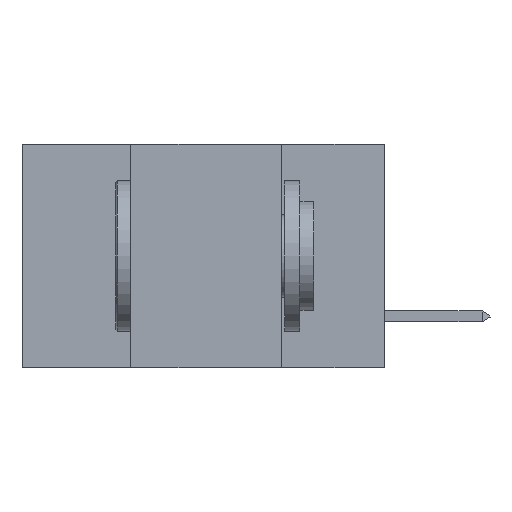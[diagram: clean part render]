
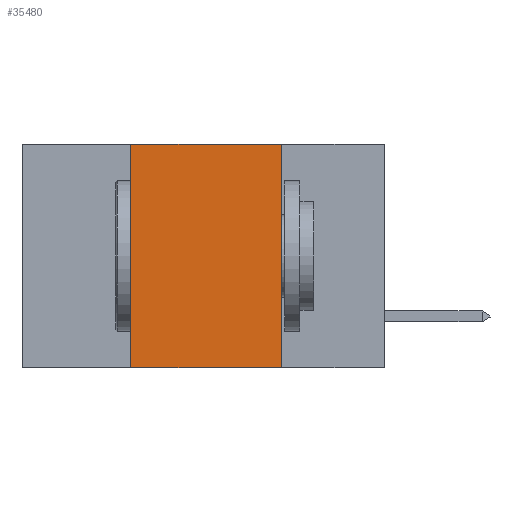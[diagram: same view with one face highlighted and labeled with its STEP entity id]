
A CAD part, left-side view. The second image highlights one B-rep face of the part: STEP entity #35480.
In plain terms, the highlighted planar face has unit normal (-1, 0, 0).
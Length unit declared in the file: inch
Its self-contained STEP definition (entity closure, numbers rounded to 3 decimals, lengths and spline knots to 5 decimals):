
#1150 = CARTESIAN_POINT ( 'NONE',  ( 0., 0.17, -0.37 ) ) ;
#1853 = CARTESIAN_POINT ( 'NONE',  ( 0., 0.42, 0. ) ) ;
#5562 = ORIENTED_EDGE ( 'NONE', *, *, #40684, .F. ) ;
#9943 = VECTOR ( 'NONE', #13408, 39.37008 ) ;
#10858 = DIRECTION ( 'NONE',  ( 0., -1., 0. ) ) ;
#11159 = ORIENTED_EDGE ( 'NONE', *, *, #45193, .T. ) ;
#12161 = DIRECTION ( 'NONE',  ( 0., -1., 0. ) ) ;
#12450 = EDGE_LOOP ( 'NONE', ( #5562, #14109, #42542, #11159 ) ) ;
#12454 = LINE ( 'NONE', #26437, #38988 ) ;
#12460 = CARTESIAN_POINT ( 'NONE',  ( 0., 0.6, 0. ) ) ;
#12589 = VERTEX_POINT ( 'NONE', #1150 ) ;
#13408 = DIRECTION ( 'NONE',  ( 0., 0., 1. ) ) ;
#13630 = VECTOR ( 'NONE', #12161, 39.37008 ) ;
#14109 = ORIENTED_EDGE ( 'NONE', *, *, #49645, .F. ) ;
#15877 = FACE_OUTER_BOUND ( 'NONE', #12450, .T. ) ;
#19212 = LINE ( 'NONE', #19946, #13630 ) ;
#19946 = CARTESIAN_POINT ( 'NONE',  ( 0., 0.6, -0.37 ) ) ;
#21953 = AXIS2_PLACEMENT_3D ( 'NONE', #12460, #40065, #24423 ) ;
#24423 = DIRECTION ( 'NONE',  ( 0., 0., -1. ) ) ;
#24601 = LINE ( 'NONE', #28162, #37528 ) ;
#26326 = VERTEX_POINT ( 'NONE', #37437 ) ;
#26437 = CARTESIAN_POINT ( 'NONE',  ( 0., 0.6, 0. ) ) ;
#28162 = CARTESIAN_POINT ( 'NONE',  ( 0., 0.17, 0. ) ) ;
#35480 = ADVANCED_FACE ( 'NONE', ( #15877 ), #36307, .F. ) ;
#36307 = PLANE ( 'NONE',  #21953 ) ;
#36536 = CARTESIAN_POINT ( 'NONE',  ( 0., 0.17, 0. ) ) ;
#37437 = CARTESIAN_POINT ( 'NONE',  ( 0., 0.42, 0. ) ) ;
#37528 = VECTOR ( 'NONE', #39824, 39.37008 ) ;
#38988 = VECTOR ( 'NONE', #10858, 39.37008 ) ;
#39824 = DIRECTION ( 'NONE',  ( 0., 0., -1. ) ) ;
#40065 = DIRECTION ( 'NONE',  ( 1., 0., 0. ) ) ;
#40684 = EDGE_CURVE ( 'NONE', #46856, #12589, #24601, .T. ) ;
#40964 = VERTEX_POINT ( 'NONE', #49259 ) ;
#42542 = ORIENTED_EDGE ( 'NONE', *, *, #50031, .F. ) ;
#45193 = EDGE_CURVE ( 'NONE', #40964, #12589, #19212, .T. ) ;
#46856 = VERTEX_POINT ( 'NONE', #36536 ) ;
#48759 = LINE ( 'NONE', #1853, #9943 ) ;
#49259 = CARTESIAN_POINT ( 'NONE',  ( 0., 0.42, -0.37 ) ) ;
#49645 = EDGE_CURVE ( 'NONE', #26326, #46856, #12454, .T. ) ;
#50031 = EDGE_CURVE ( 'NONE', #40964, #26326, #48759, .T. ) ;
